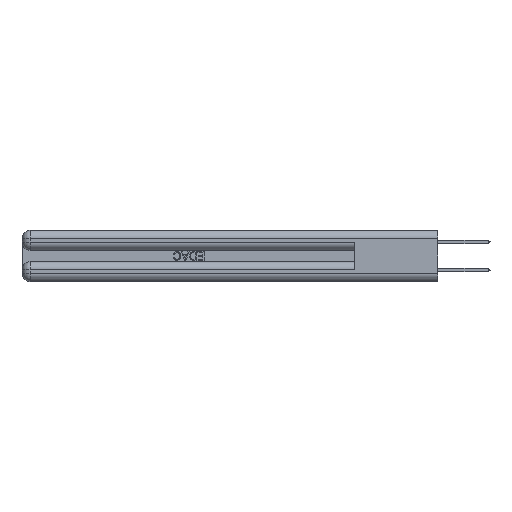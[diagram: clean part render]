
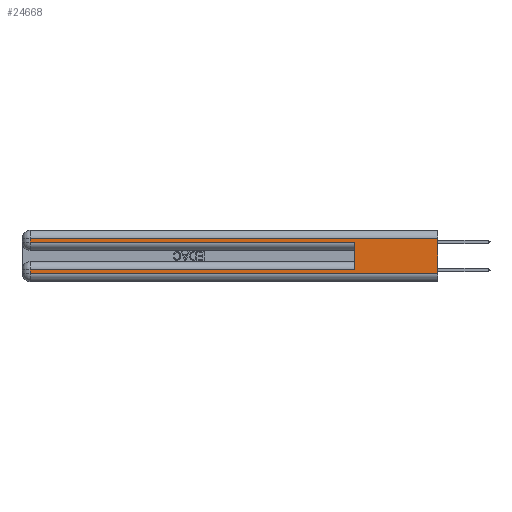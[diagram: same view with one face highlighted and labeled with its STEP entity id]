
A CAD part, left-side view. The second image highlights one B-rep face of the part: STEP entity #24668.
In plain terms, the highlighted planar face has unit normal (-1, 0, 0).
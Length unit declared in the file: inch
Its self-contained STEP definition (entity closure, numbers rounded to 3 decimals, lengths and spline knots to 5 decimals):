
#68 = CARTESIAN_POINT ( 'NONE',  ( 0., 0., 0.06 ) ) ;
#797 = FACE_OUTER_BOUND ( 'NONE', #15433, .T. ) ;
#1613 = CARTESIAN_POINT ( 'NONE',  ( 0., 2.94, 0.37 ) ) ;
#2374 = CARTESIAN_POINT ( 'NONE',  ( 0., 2.94, 0.37 ) ) ;
#2624 = CARTESIAN_POINT ( 'NONE',  ( 0., 0., 0.285 ) ) ;
#2856 = CARTESIAN_POINT ( 'NONE',  ( 0., 0.6, 0.085 ) ) ;
#4215 = VERTEX_POINT ( 'NONE', #68 ) ;
#4294 = CARTESIAN_POINT ( 'NONE',  ( 0., 2.94, 0.06 ) ) ;
#4732 = EDGE_CURVE ( 'NONE', #23452, #24015, #15248, .T. ) ;
#4832 = ORIENTED_EDGE ( 'NONE', *, *, #24403, .T. ) ;
#5102 = LINE ( 'NONE', #1613, #12985 ) ;
#6904 = VECTOR ( 'NONE', #8609, 39.37008 ) ;
#7834 = LINE ( 'NONE', #11592, #6904 ) ;
#7896 = CARTESIAN_POINT ( 'NONE',  ( 0., 0., 0.31 ) ) ;
#7962 = CARTESIAN_POINT ( 'NONE',  ( 0., 2.94, 0.31 ) ) ;
#8519 = CARTESIAN_POINT ( 'NONE',  ( 0., 0.6, 0.285 ) ) ;
#8609 = DIRECTION ( 'NONE',  ( 0., 0., 1. ) ) ;
#8631 = DIRECTION ( 'NONE',  ( 0., -1., 0. ) ) ;
#8787 = ORIENTED_EDGE ( 'NONE', *, *, #26786, .T. ) ;
#8949 = VECTOR ( 'NONE', #31394, 39.37008 ) ;
#9443 = ORIENTED_EDGE ( 'NONE', *, *, #11104, .T. ) ;
#10212 = LINE ( 'NONE', #34011, #32696 ) ;
#10370 = PLANE ( 'NONE',  #28917 ) ;
#11104 = EDGE_CURVE ( 'NONE', #25169, #19981, #17652, .T. ) ;
#11592 = CARTESIAN_POINT ( 'NONE',  ( 0., 0.6, 0.145 ) ) ;
#12151 = CARTESIAN_POINT ( 'NONE',  ( 0., 0., 0.31 ) ) ;
#12985 = VECTOR ( 'NONE', #16366, 39.37008 ) ;
#13850 = VERTEX_POINT ( 'NONE', #2856 ) ;
#15248 = LINE ( 'NONE', #2374, #36849 ) ;
#15433 = EDGE_LOOP ( 'NONE', ( #37033, #9443, #37282, #8787, #35181, #4832, #33404, #30169 ) ) ;
#15713 = VERTEX_POINT ( 'NONE', #27722 ) ;
#16366 = DIRECTION ( 'NONE',  ( 0., 0., -1. ) ) ;
#17006 = LINE ( 'NONE', #26388, #32645 ) ;
#17642 = EDGE_CURVE ( 'NONE', #25169, #4215, #38099, .T. ) ;
#17652 = LINE ( 'NONE', #7896, #8949 ) ;
#17655 = DIRECTION ( 'NONE',  ( 0., 1., 0. ) ) ;
#19182 = DIRECTION ( 'NONE',  ( 0., 0., -1. ) ) ;
#19981 = VERTEX_POINT ( 'NONE', #7962 ) ;
#22768 = EDGE_CURVE ( 'NONE', #19981, #15713, #5102, .T. ) ;
#22781 = VECTOR ( 'NONE', #8631, 39.37008 ) ;
#22995 = DIRECTION ( 'NONE',  ( 0., 0., -1. ) ) ;
#23369 = VECTOR ( 'NONE', #31548, 39.37008 ) ;
#23452 = VERTEX_POINT ( 'NONE', #34424 ) ;
#23606 = EDGE_CURVE ( 'NONE', #13850, #36322, #7834, .T. ) ;
#24015 = VERTEX_POINT ( 'NONE', #4294 ) ;
#24403 = EDGE_CURVE ( 'NONE', #13850, #23452, #17006, .T. ) ;
#24668 = ADVANCED_FACE ( 'NONE', ( #797 ), #10370, .F. ) ;
#25169 = VERTEX_POINT ( 'NONE', #12151 ) ;
#26388 = CARTESIAN_POINT ( 'NONE',  ( 0., 0., 0.085 ) ) ;
#26786 = EDGE_CURVE ( 'NONE', #15713, #36322, #30634, .T. ) ;
#27722 = CARTESIAN_POINT ( 'NONE',  ( 0., 2.94, 0.285 ) ) ;
#27934 = CARTESIAN_POINT ( 'NONE',  ( 0., 0., 0.37 ) ) ;
#28584 = CARTESIAN_POINT ( 'NONE',  ( 0., 0., 0.37 ) ) ;
#28917 = AXIS2_PLACEMENT_3D ( 'NONE', #27934, #36804, #19182 ) ;
#30169 = ORIENTED_EDGE ( 'NONE', *, *, #35649, .T. ) ;
#30634 = LINE ( 'NONE', #2624, #22781 ) ;
#31394 = DIRECTION ( 'NONE',  ( 0., 1., 0. ) ) ;
#31548 = DIRECTION ( 'NONE',  ( 0., 0., -1. ) ) ;
#32645 = VECTOR ( 'NONE', #17655, 39.37008 ) ;
#32696 = VECTOR ( 'NONE', #36980, 39.37008 ) ;
#33404 = ORIENTED_EDGE ( 'NONE', *, *, #4732, .T. ) ;
#34011 = CARTESIAN_POINT ( 'NONE',  ( 0., 0., 0.06 ) ) ;
#34424 = CARTESIAN_POINT ( 'NONE',  ( 0., 2.94, 0.085 ) ) ;
#35181 = ORIENTED_EDGE ( 'NONE', *, *, #23606, .F. ) ;
#35649 = EDGE_CURVE ( 'NONE', #24015, #4215, #10212, .T. ) ;
#36322 = VERTEX_POINT ( 'NONE', #8519 ) ;
#36804 = DIRECTION ( 'NONE',  ( 1., 0., 0. ) ) ;
#36849 = VECTOR ( 'NONE', #22995, 39.37008 ) ;
#36980 = DIRECTION ( 'NONE',  ( 0., -1., 0. ) ) ;
#37033 = ORIENTED_EDGE ( 'NONE', *, *, #17642, .F. ) ;
#37282 = ORIENTED_EDGE ( 'NONE', *, *, #22768, .T. ) ;
#38099 = LINE ( 'NONE', #28584, #23369 ) ;
